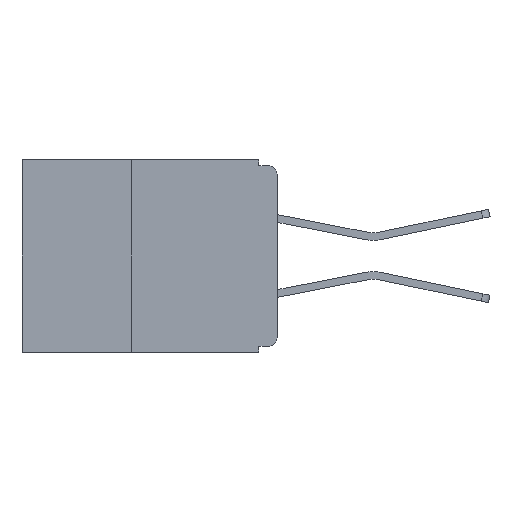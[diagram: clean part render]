
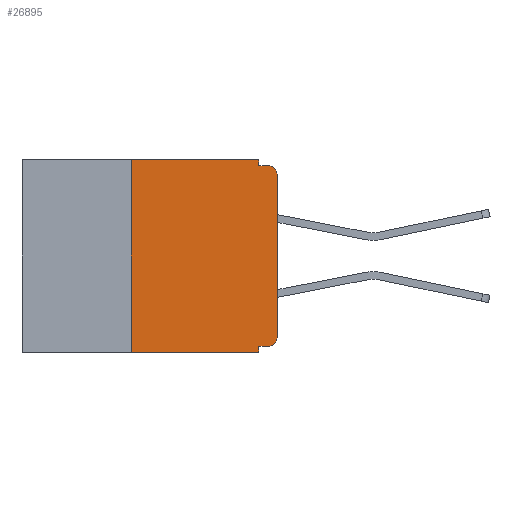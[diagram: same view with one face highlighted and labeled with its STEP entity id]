
A CAD part, left-side view. The second image highlights one B-rep face of the part: STEP entity #26895.
In plain terms, the highlighted planar face has unit normal (-1, 0, 0).
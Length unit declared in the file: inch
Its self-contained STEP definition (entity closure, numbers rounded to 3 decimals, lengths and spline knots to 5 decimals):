
#877 = DIRECTION ( 'NONE',  ( 0., 0., -1. ) ) ;
#932 = ORIENTED_EDGE ( 'NONE', *, *, #17223, .F. ) ;
#1445 = CARTESIAN_POINT ( 'NONE',  ( 0., 0.031, 0. ) ) ;
#1722 = PLANE ( 'NONE',  #22465 ) ;
#1905 = AXIS2_PLACEMENT_3D ( 'NONE', #7074, #21763, #9184 ) ;
#2147 = ORIENTED_EDGE ( 'NONE', *, *, #4415, .T. ) ;
#2216 = DIRECTION ( 'NONE',  ( 0., -1., 0. ) ) ;
#2774 = VERTEX_POINT ( 'NONE', #17599 ) ;
#2824 = VERTEX_POINT ( 'NONE', #14501 ) ;
#3192 = LINE ( 'NONE', #14717, #8249 ) ;
#3847 = CARTESIAN_POINT ( 'NONE',  ( 0., 0.437, 0. ) ) ;
#3882 = VECTOR ( 'NONE', #877, 39.37008 ) ;
#4414 = DIRECTION ( 'NONE',  ( 0., 0., 1. ) ) ;
#4415 = EDGE_CURVE ( 'NONE', #8764, #22177, #15811, .T. ) ;
#4468 = DIRECTION ( 'NONE',  ( 0., 0., 1. ) ) ;
#4510 = LINE ( 'NONE', #17179, #21358 ) ;
#4828 = EDGE_LOOP ( 'NONE', ( #18555, #7379, #5901, #8274, #932, #18988, #2147, #20171, #17922, #23626 ) ) ;
#5293 = VECTOR ( 'NONE', #2216, 39.37008 ) ;
#5901 = ORIENTED_EDGE ( 'NONE', *, *, #15809, .F. ) ;
#6889 = CARTESIAN_POINT ( 'NONE',  ( 0., 0.25, 0. ) ) ;
#7074 = CARTESIAN_POINT ( 'NONE',  ( 0., 0.015, -0.025 ) ) ;
#7344 = VECTOR ( 'NONE', #17536, 39.37008 ) ;
#7379 = ORIENTED_EDGE ( 'NONE', *, *, #23298, .T. ) ;
#7981 = AXIS2_PLACEMENT_3D ( 'NONE', #24312, #11774, #26387 ) ;
#8167 = CARTESIAN_POINT ( 'NONE',  ( 0., 0.031, -0.01 ) ) ;
#8202 = DIRECTION ( 'NONE',  ( 1., 0., 0. ) ) ;
#8249 = VECTOR ( 'NONE', #16839, 39.37008 ) ;
#8274 = ORIENTED_EDGE ( 'NONE', *, *, #15285, .F. ) ;
#8527 = CIRCLE ( 'NONE', #7981, 0.015 ) ;
#8764 = VERTEX_POINT ( 'NONE', #12148 ) ;
#9184 = DIRECTION ( 'NONE',  ( 0., 0., -1. ) ) ;
#9234 = CARTESIAN_POINT ( 'NONE',  ( 0., 0.031, -0.33 ) ) ;
#10014 = CARTESIAN_POINT ( 'NONE',  ( 0., 0.015, -0.32 ) ) ;
#10305 = VERTEX_POINT ( 'NONE', #20897 ) ;
#10409 = EDGE_CURVE ( 'NONE', #2774, #23060, #4510, .T. ) ;
#11221 = CARTESIAN_POINT ( 'NONE',  ( 0., 0.031, 0. ) ) ;
#11313 = VERTEX_POINT ( 'NONE', #1445 ) ;
#11394 = EDGE_CURVE ( 'NONE', #17114, #2824, #24913, .T. ) ;
#11577 = EDGE_CURVE ( 'NONE', #8764, #19462, #26494, .T. ) ;
#11774 = DIRECTION ( 'NONE',  ( -1., 0., 0. ) ) ;
#12148 = CARTESIAN_POINT ( 'NONE',  ( 0., 0.25, -0.33 ) ) ;
#12399 = CIRCLE ( 'NONE', #1905, 0.015 ) ;
#12916 = CARTESIAN_POINT ( 'NONE',  ( 0., 0., -0.01 ) ) ;
#12971 = LINE ( 'NONE', #11221, #7344 ) ;
#13527 = CARTESIAN_POINT ( 'NONE',  ( 0., 0.437, -0.33 ) ) ;
#14192 = FACE_OUTER_BOUND ( 'NONE', #4828, .T. ) ;
#14501 = CARTESIAN_POINT ( 'NONE',  ( 0., 0.031, -0.32 ) ) ;
#14544 = DIRECTION ( 'NONE',  ( 0., -1., 0. ) ) ;
#14717 = CARTESIAN_POINT ( 'NONE',  ( 0., 0.437, 0. ) ) ;
#14759 = VECTOR ( 'NONE', #4414, 39.37008 ) ;
#15104 = VERTEX_POINT ( 'NONE', #8167 ) ;
#15285 = EDGE_CURVE ( 'NONE', #11313, #15104, #12971, .T. ) ;
#15670 = CARTESIAN_POINT ( 'NONE',  ( 0., 0.031, -0.33 ) ) ;
#15809 = EDGE_CURVE ( 'NONE', #15104, #10305, #22093, .T. ) ;
#15811 = LINE ( 'NONE', #13527, #21356 ) ;
#16579 = CARTESIAN_POINT ( 'NONE',  ( 0., 0., -0.32 ) ) ;
#16839 = DIRECTION ( 'NONE',  ( 0., -1., 0. ) ) ;
#17114 = VERTEX_POINT ( 'NONE', #10014 ) ;
#17132 = CARTESIAN_POINT ( 'NONE',  ( 0., 0.25, -0.33 ) ) ;
#17179 = CARTESIAN_POINT ( 'NONE',  ( 0., 0., 0. ) ) ;
#17223 = EDGE_CURVE ( 'NONE', #19462, #11313, #3192, .T. ) ;
#17536 = DIRECTION ( 'NONE',  ( 0., 0., -1. ) ) ;
#17599 = CARTESIAN_POINT ( 'NONE',  ( 0., 0., -0.305 ) ) ;
#17922 = ORIENTED_EDGE ( 'NONE', *, *, #11394, .F. ) ;
#18409 = CARTESIAN_POINT ( 'NONE',  ( 0., 0., -0.025 ) ) ;
#18555 = ORIENTED_EDGE ( 'NONE', *, *, #10409, .T. ) ;
#18988 = ORIENTED_EDGE ( 'NONE', *, *, #11577, .F. ) ;
#19462 = VERTEX_POINT ( 'NONE', #6889 ) ;
#19981 = VECTOR ( 'NONE', #26905, 39.37008 ) ;
#20171 = ORIENTED_EDGE ( 'NONE', *, *, #26639, .F. ) ;
#20897 = CARTESIAN_POINT ( 'NONE',  ( 0., 0.015, -0.01 ) ) ;
#21356 = VECTOR ( 'NONE', #14544, 39.37008 ) ;
#21358 = VECTOR ( 'NONE', #4468, 39.37008 ) ;
#21407 = LINE ( 'NONE', #15670, #3882 ) ;
#21684 = EDGE_CURVE ( 'NONE', #17114, #2774, #8527, .T. ) ;
#21763 = DIRECTION ( 'NONE',  ( -1., 0., 0. ) ) ;
#22093 = LINE ( 'NONE', #12916, #5293 ) ;
#22177 = VERTEX_POINT ( 'NONE', #9234 ) ;
#22465 = AXIS2_PLACEMENT_3D ( 'NONE', #3847, #8202, #22870 ) ;
#22870 = DIRECTION ( 'NONE',  ( 0., 0., -1. ) ) ;
#23060 = VERTEX_POINT ( 'NONE', #18409 ) ;
#23298 = EDGE_CURVE ( 'NONE', #23060, #10305, #12399, .T. ) ;
#23626 = ORIENTED_EDGE ( 'NONE', *, *, #21684, .T. ) ;
#24312 = CARTESIAN_POINT ( 'NONE',  ( 0., 0.015, -0.305 ) ) ;
#24913 = LINE ( 'NONE', #16579, #19981 ) ;
#26387 = DIRECTION ( 'NONE',  ( 0., 0., -1. ) ) ;
#26494 = LINE ( 'NONE', #17132, #14759 ) ;
#26639 = EDGE_CURVE ( 'NONE', #2824, #22177, #21407, .T. ) ;
#26895 = ADVANCED_FACE ( 'NONE', ( #14192 ), #1722, .F. ) ;
#26905 = DIRECTION ( 'NONE',  ( 0., 1., 0. ) ) ;
